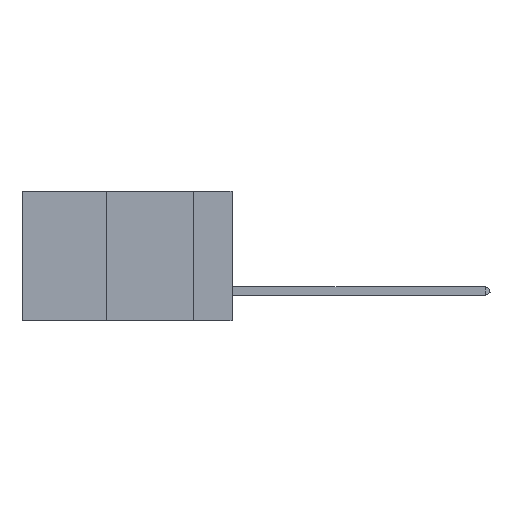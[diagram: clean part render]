
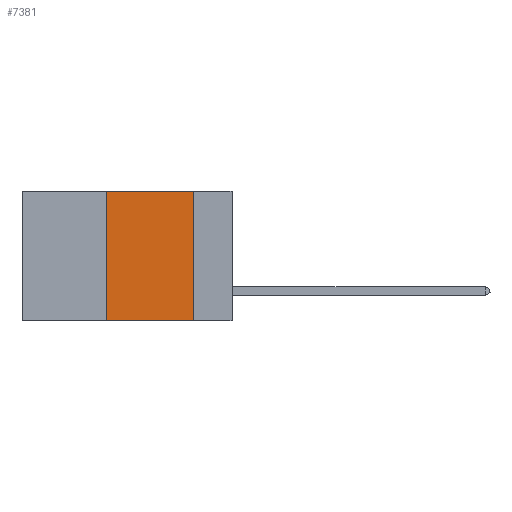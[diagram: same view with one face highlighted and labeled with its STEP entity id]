
A CAD part, left-side view. The second image highlights one B-rep face of the part: STEP entity #7381.
In plain terms, the highlighted planar face has unit normal (-1, 0, 0).
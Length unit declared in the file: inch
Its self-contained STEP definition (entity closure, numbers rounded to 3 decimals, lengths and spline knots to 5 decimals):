
#177 = DIRECTION ( 'NONE',  ( 0., -1., 0. ) ) ;
#382 = LINE ( 'NONE', #13013, #4775 ) ;
#1318 = EDGE_CURVE ( 'NONE', #13795, #11710, #6242, .T. ) ;
#1665 = CARTESIAN_POINT ( 'NONE',  ( 0., 0.36, 0. ) ) ;
#2008 = EDGE_LOOP ( 'NONE', ( #2610, #14655, #4805, #5066 ) ) ;
#2188 = EDGE_CURVE ( 'NONE', #3080, #13795, #14696, .T. ) ;
#2313 = CARTESIAN_POINT ( 'NONE',  ( 0., 0.36, 0. ) ) ;
#2610 = ORIENTED_EDGE ( 'NONE', *, *, #14799, .F. ) ;
#2720 = CARTESIAN_POINT ( 'NONE',  ( 0., 0.36, -0.37 ) ) ;
#3080 = VERTEX_POINT ( 'NONE', #2720 ) ;
#4336 = EDGE_CURVE ( 'NONE', #3080, #13051, #5335, .T. ) ;
#4775 = VECTOR ( 'NONE', #10237, 39.37008 ) ;
#4805 = ORIENTED_EDGE ( 'NONE', *, *, #2188, .F. ) ;
#4941 = DIRECTION ( 'NONE',  ( 0., 0., 1. ) ) ;
#5066 = ORIENTED_EDGE ( 'NONE', *, *, #4336, .T. ) ;
#5335 = LINE ( 'NONE', #15981, #15045 ) ;
#6242 = LINE ( 'NONE', #15598, #10276 ) ;
#6795 = VECTOR ( 'NONE', #4941, 39.37008 ) ;
#7381 = ADVANCED_FACE ( 'NONE', ( #9008 ), #13706, .F. ) ;
#8354 = DIRECTION ( 'NONE',  ( 0., 0., -1. ) ) ;
#8578 = CARTESIAN_POINT ( 'NONE',  ( 0., 0.6, 0. ) ) ;
#9008 = FACE_OUTER_BOUND ( 'NONE', #2008, .T. ) ;
#9758 = AXIS2_PLACEMENT_3D ( 'NONE', #8578, #16091, #8354 ) ;
#10066 = DIRECTION ( 'NONE',  ( 0., -1., 0. ) ) ;
#10237 = DIRECTION ( 'NONE',  ( 0., 0., -1. ) ) ;
#10276 = VECTOR ( 'NONE', #177, 39.37008 ) ;
#11480 = CARTESIAN_POINT ( 'NONE',  ( 0., 0.11, 0. ) ) ;
#11710 = VERTEX_POINT ( 'NONE', #11480 ) ;
#11815 = CARTESIAN_POINT ( 'NONE',  ( 0., 0.11, -0.37 ) ) ;
#13013 = CARTESIAN_POINT ( 'NONE',  ( 0., 0.11, 0. ) ) ;
#13051 = VERTEX_POINT ( 'NONE', #11815 ) ;
#13706 = PLANE ( 'NONE',  #9758 ) ;
#13795 = VERTEX_POINT ( 'NONE', #1665 ) ;
#14655 = ORIENTED_EDGE ( 'NONE', *, *, #1318, .F. ) ;
#14696 = LINE ( 'NONE', #2313, #6795 ) ;
#14799 = EDGE_CURVE ( 'NONE', #11710, #13051, #382, .T. ) ;
#15045 = VECTOR ( 'NONE', #10066, 39.37008 ) ;
#15598 = CARTESIAN_POINT ( 'NONE',  ( 0., 0.6, 0. ) ) ;
#15981 = CARTESIAN_POINT ( 'NONE',  ( 0., 0.6, -0.37 ) ) ;
#16091 = DIRECTION ( 'NONE',  ( 1., 0., 0. ) ) ;
